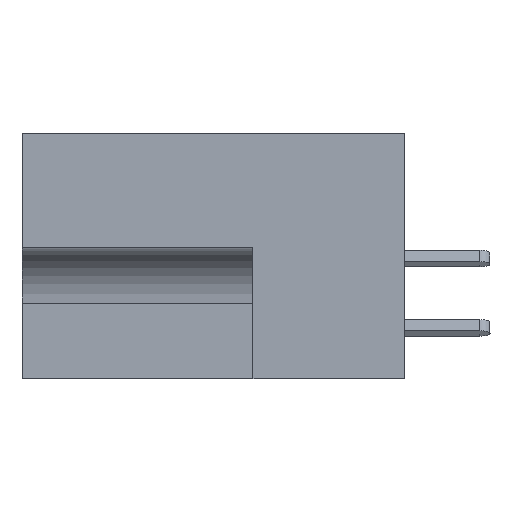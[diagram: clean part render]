
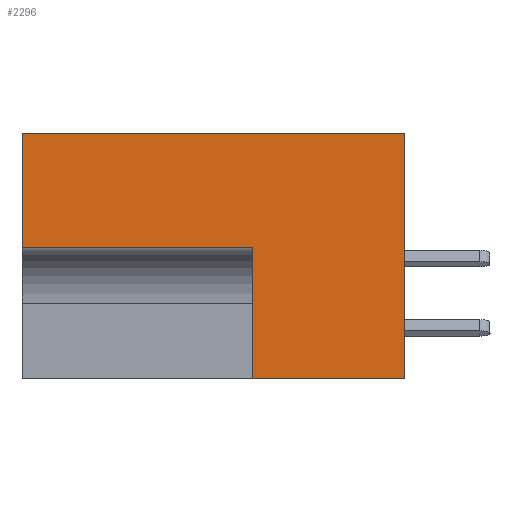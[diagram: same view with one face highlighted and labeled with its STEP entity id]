
A CAD part, left-side view. The second image highlights one B-rep face of the part: STEP entity #2296.
In plain terms, the highlighted planar face has unit normal (-1, 0, 0).
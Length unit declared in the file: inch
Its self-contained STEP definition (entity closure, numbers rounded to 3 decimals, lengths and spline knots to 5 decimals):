
#400 = DIRECTION ( 'NONE',  ( 0., 0., 1. ) ) ;
#801 = CARTESIAN_POINT ( 'NONE',  ( 0., 0.828, -0.248 ) ) ;
#913 = VERTEX_POINT ( 'NONE', #801 ) ;
#1153 = CARTESIAN_POINT ( 'NONE',  ( 0., 0., 0. ) ) ;
#1590 = VERTEX_POINT ( 'NONE', #25383 ) ;
#1834 = EDGE_CURVE ( 'NONE', #9946, #1590, #24268, .T. ) ;
#2296 = ADVANCED_FACE ( 'NONE', ( #26666 ), #19412, .F. ) ;
#2709 = LINE ( 'NONE', #20159, #16634 ) ;
#3911 = LINE ( 'NONE', #6247, #9328 ) ;
#5940 = VECTOR ( 'NONE', #17966, 39.37008 ) ;
#6121 = CARTESIAN_POINT ( 'NONE',  ( 0., 0.328, -0.531 ) ) ;
#6247 = CARTESIAN_POINT ( 'NONE',  ( 0., 0.453, 0. ) ) ;
#6257 = LINE ( 'NONE', #23178, #17880 ) ;
#6267 = DIRECTION ( 'NONE',  ( 1., 0., 0. ) ) ;
#6539 = CARTESIAN_POINT ( 'NONE',  ( 0., 0.828, 0. ) ) ;
#6978 = EDGE_CURVE ( 'NONE', #21322, #16088, #3911, .T. ) ;
#7345 = CARTESIAN_POINT ( 'NONE',  ( 0., 0.328, -0.531 ) ) ;
#8109 = ORIENTED_EDGE ( 'NONE', *, *, #14558, .F. ) ;
#8632 = CARTESIAN_POINT ( 'NONE',  ( 0., 0.453, 0. ) ) ;
#9328 = VECTOR ( 'NONE', #10592, 39.37008 ) ;
#9946 = VERTEX_POINT ( 'NONE', #6121 ) ;
#10592 = DIRECTION ( 'NONE',  ( 0., -1., 0. ) ) ;
#11081 = ORIENTED_EDGE ( 'NONE', *, *, #1834, .F. ) ;
#12505 = EDGE_CURVE ( 'NONE', #913, #21322, #2709, .T. ) ;
#13097 = LINE ( 'NONE', #26400, #5940 ) ;
#13268 = AXIS2_PLACEMENT_3D ( 'NONE', #8632, #6267, #26126 ) ;
#14558 = EDGE_CURVE ( 'NONE', #1590, #913, #13097, .T. ) ;
#14591 = DIRECTION ( 'NONE',  ( 0., -1., 0. ) ) ;
#16088 = VERTEX_POINT ( 'NONE', #27942 ) ;
#16373 = DIRECTION ( 'NONE',  ( 0., 0., 1. ) ) ;
#16388 = EDGE_CURVE ( 'NONE', #24546, #16088, #17764, .T. ) ;
#16634 = VECTOR ( 'NONE', #400, 39.37008 ) ;
#17074 = CARTESIAN_POINT ( 'NONE',  ( 0., 0., -0.531 ) ) ;
#17764 = LINE ( 'NONE', #1153, #27339 ) ;
#17880 = VECTOR ( 'NONE', #14591, 39.37008 ) ;
#17966 = DIRECTION ( 'NONE',  ( 0., 1., 0. ) ) ;
#18112 = ORIENTED_EDGE ( 'NONE', *, *, #20380, .T. ) ;
#18413 = DIRECTION ( 'NONE',  ( 0., 0., 1. ) ) ;
#19412 = PLANE ( 'NONE',  #13268 ) ;
#19422 = EDGE_LOOP ( 'NONE', ( #24002, #8109, #11081, #18112, #22986, #26428 ) ) ;
#20159 = CARTESIAN_POINT ( 'NONE',  ( 0., 0.828, 0. ) ) ;
#20380 = EDGE_CURVE ( 'NONE', #9946, #24546, #6257, .T. ) ;
#21322 = VERTEX_POINT ( 'NONE', #6539 ) ;
#22986 = ORIENTED_EDGE ( 'NONE', *, *, #16388, .T. ) ;
#23178 = CARTESIAN_POINT ( 'NONE',  ( 0., 0.453, -0.531 ) ) ;
#23922 = VECTOR ( 'NONE', #18413, 39.37008 ) ;
#24002 = ORIENTED_EDGE ( 'NONE', *, *, #12505, .F. ) ;
#24268 = LINE ( 'NONE', #7345, #23922 ) ;
#24546 = VERTEX_POINT ( 'NONE', #17074 ) ;
#25383 = CARTESIAN_POINT ( 'NONE',  ( 0., 0.328, -0.248 ) ) ;
#26126 = DIRECTION ( 'NONE',  ( 0., 0., -1. ) ) ;
#26400 = CARTESIAN_POINT ( 'NONE',  ( 0., 0.328, -0.248 ) ) ;
#26428 = ORIENTED_EDGE ( 'NONE', *, *, #6978, .F. ) ;
#26666 = FACE_OUTER_BOUND ( 'NONE', #19422, .T. ) ;
#27339 = VECTOR ( 'NONE', #16373, 39.37008 ) ;
#27942 = CARTESIAN_POINT ( 'NONE',  ( 0., 0., 0. ) ) ;
